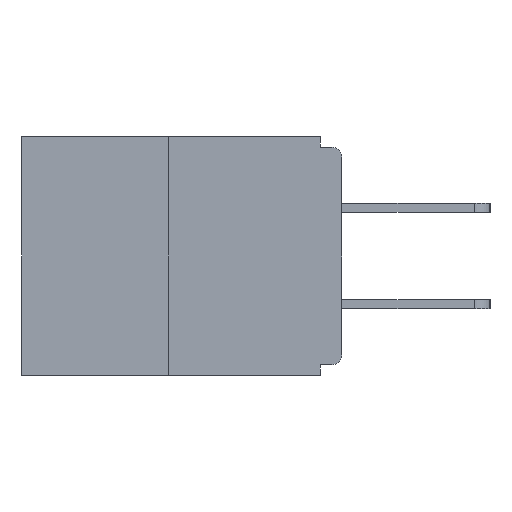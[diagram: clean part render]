
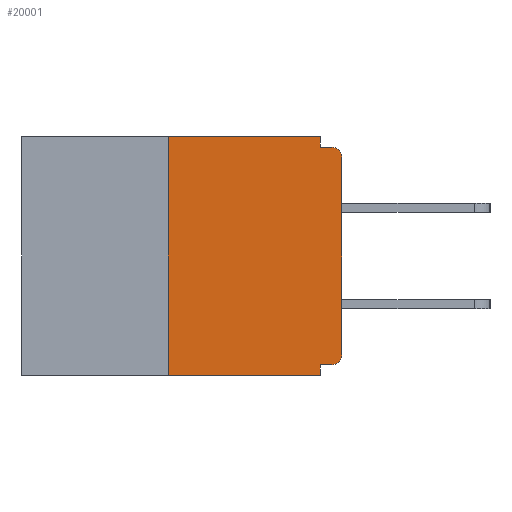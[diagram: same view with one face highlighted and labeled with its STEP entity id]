
A CAD part, left-side view. The second image highlights one B-rep face of the part: STEP entity #20001.
In plain terms, the highlighted planar face has unit normal (-1, 0, 0).
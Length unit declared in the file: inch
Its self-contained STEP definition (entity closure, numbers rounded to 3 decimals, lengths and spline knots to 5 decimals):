
#694 = CARTESIAN_POINT ( 'NONE',  ( 0., 0.031, -0.328 ) ) ;
#974 = CIRCLE ( 'NONE', #20030, 0.015 ) ;
#2123 = CARTESIAN_POINT ( 'NONE',  ( 0., 0., -0.03 ) ) ;
#2350 = LINE ( 'NONE', #13186, #14965 ) ;
#2419 = DIRECTION ( 'NONE',  ( 0., 0., 1. ) ) ;
#2422 = EDGE_CURVE ( 'NONE', #6759, #5591, #13960, .T. ) ;
#2708 = EDGE_CURVE ( 'NONE', #6008, #3499, #16280, .T. ) ;
#2768 = DIRECTION ( 'NONE',  ( 0., 0., 1. ) ) ;
#2793 = EDGE_CURVE ( 'NONE', #4504, #5591, #8411, .T. ) ;
#3046 = CARTESIAN_POINT ( 'NONE',  ( 0., 0., -0.313 ) ) ;
#3499 = VERTEX_POINT ( 'NONE', #15498 ) ;
#3586 = LINE ( 'NONE', #21746, #20382 ) ;
#3905 = CIRCLE ( 'NONE', #19775, 0.015 ) ;
#4391 = CARTESIAN_POINT ( 'NONE',  ( 0., 0.25, 0. ) ) ;
#4504 = VERTEX_POINT ( 'NONE', #14074 ) ;
#4991 = DIRECTION ( 'NONE',  ( 0., 0., -1. ) ) ;
#5195 = DIRECTION ( 'NONE',  ( 0., 0., -1. ) ) ;
#5329 = EDGE_CURVE ( 'NONE', #3499, #14498, #3586, .T. ) ;
#5591 = VERTEX_POINT ( 'NONE', #10942 ) ;
#5927 = AXIS2_PLACEMENT_3D ( 'NONE', #21095, #7773, #10938 ) ;
#6008 = VERTEX_POINT ( 'NONE', #6729 ) ;
#6123 = CARTESIAN_POINT ( 'NONE',  ( 0., 0.015, -0.015 ) ) ;
#6729 = CARTESIAN_POINT ( 'NONE',  ( 0., 0.25, 0. ) ) ;
#6759 = VERTEX_POINT ( 'NONE', #694 ) ;
#6825 = DIRECTION ( 'NONE',  ( 0., 0., -1. ) ) ;
#7468 = VERTEX_POINT ( 'NONE', #10617 ) ;
#7773 = DIRECTION ( 'NONE',  ( 1., 0., 0. ) ) ;
#7795 = CARTESIAN_POINT ( 'NONE',  ( 0., 0.015, -0.313 ) ) ;
#7820 = VERTEX_POINT ( 'NONE', #6123 ) ;
#8411 = LINE ( 'NONE', #15099, #11867 ) ;
#8590 = CARTESIAN_POINT ( 'NONE',  ( 0., 0.015, -0.03 ) ) ;
#8704 = VERTEX_POINT ( 'NONE', #2123 ) ;
#8822 = EDGE_CURVE ( 'NONE', #14498, #7820, #2350, .T. ) ;
#8902 = EDGE_CURVE ( 'NONE', #4504, #6008, #9736, .T. ) ;
#9533 = EDGE_CURVE ( 'NONE', #7468, #18814, #974, .T. ) ;
#9736 = LINE ( 'NONE', #4391, #16296 ) ;
#9774 = CARTESIAN_POINT ( 'NONE',  ( 0., 0.031, -0.015 ) ) ;
#9923 = EDGE_CURVE ( 'NONE', #18814, #8704, #11828, .T. ) ;
#10279 = DIRECTION ( 'NONE',  ( -1., 0., 0. ) ) ;
#10617 = CARTESIAN_POINT ( 'NONE',  ( 0., 0.015, -0.328 ) ) ;
#10938 = DIRECTION ( 'NONE',  ( 0., 0., -1. ) ) ;
#10942 = CARTESIAN_POINT ( 'NONE',  ( 0., 0.031, -0.343 ) ) ;
#11587 = ORIENTED_EDGE ( 'NONE', *, *, #8822, .F. ) ;
#11828 = LINE ( 'NONE', #20827, #21231 ) ;
#11867 = VECTOR ( 'NONE', #18313, 39.37008 ) ;
#11904 = ORIENTED_EDGE ( 'NONE', *, *, #17702, .T. ) ;
#13186 = CARTESIAN_POINT ( 'NONE',  ( 0., 0., -0.015 ) ) ;
#13726 = ORIENTED_EDGE ( 'NONE', *, *, #9923, .T. ) ;
#13960 = LINE ( 'NONE', #18189, #14972 ) ;
#14000 = VECTOR ( 'NONE', #20328, 39.37008 ) ;
#14074 = CARTESIAN_POINT ( 'NONE',  ( 0., 0.25, -0.343 ) ) ;
#14498 = VERTEX_POINT ( 'NONE', #9774 ) ;
#14740 = CARTESIAN_POINT ( 'NONE',  ( 0., 0.46, 0. ) ) ;
#14812 = DIRECTION ( 'NONE',  ( 0., -1., 0. ) ) ;
#14965 = VECTOR ( 'NONE', #18192, 39.37008 ) ;
#14972 = VECTOR ( 'NONE', #4991, 39.37008 ) ;
#15099 = CARTESIAN_POINT ( 'NONE',  ( 0., 0.46, -0.343 ) ) ;
#15498 = CARTESIAN_POINT ( 'NONE',  ( 0., 0.031, 0. ) ) ;
#15948 = DIRECTION ( 'NONE',  ( -1., 0., 0. ) ) ;
#16061 = PLANE ( 'NONE',  #5927 ) ;
#16280 = LINE ( 'NONE', #14740, #21260 ) ;
#16296 = VECTOR ( 'NONE', #2768, 39.37008 ) ;
#16445 = ORIENTED_EDGE ( 'NONE', *, *, #5329, .F. ) ;
#16863 = ORIENTED_EDGE ( 'NONE', *, *, #21469, .F. ) ;
#17202 = ORIENTED_EDGE ( 'NONE', *, *, #9533, .T. ) ;
#17702 = EDGE_CURVE ( 'NONE', #8704, #7820, #3905, .T. ) ;
#18189 = CARTESIAN_POINT ( 'NONE',  ( 0., 0.031, -0.343 ) ) ;
#18192 = DIRECTION ( 'NONE',  ( 0., -1., 0. ) ) ;
#18313 = DIRECTION ( 'NONE',  ( 0., -1., 0. ) ) ;
#18418 = LINE ( 'NONE', #18575, #14000 ) ;
#18575 = CARTESIAN_POINT ( 'NONE',  ( 0., 0., -0.328 ) ) ;
#18691 = ORIENTED_EDGE ( 'NONE', *, *, #8902, .F. ) ;
#18768 = ORIENTED_EDGE ( 'NONE', *, *, #2793, .T. ) ;
#18814 = VERTEX_POINT ( 'NONE', #3046 ) ;
#19582 = DIRECTION ( 'NONE',  ( 0., 0., -1. ) ) ;
#19775 = AXIS2_PLACEMENT_3D ( 'NONE', #8590, #10279, #6825 ) ;
#20001 = ADVANCED_FACE ( 'NONE', ( #21361 ), #16061, .F. ) ;
#20030 = AXIS2_PLACEMENT_3D ( 'NONE', #7795, #15948, #19582 ) ;
#20236 = ORIENTED_EDGE ( 'NONE', *, *, #2422, .F. ) ;
#20328 = DIRECTION ( 'NONE',  ( 0., 1., 0. ) ) ;
#20382 = VECTOR ( 'NONE', #5195, 39.37008 ) ;
#20542 = EDGE_LOOP ( 'NONE', ( #21725, #18691, #18768, #20236, #16863, #17202, #13726, #11904, #11587, #16445 ) ) ;
#20827 = CARTESIAN_POINT ( 'NONE',  ( 0., 0., 0. ) ) ;
#21095 = CARTESIAN_POINT ( 'NONE',  ( 0., 0.46, 0. ) ) ;
#21231 = VECTOR ( 'NONE', #2419, 39.37008 ) ;
#21260 = VECTOR ( 'NONE', #14812, 39.37008 ) ;
#21361 = FACE_OUTER_BOUND ( 'NONE', #20542, .T. ) ;
#21469 = EDGE_CURVE ( 'NONE', #7468, #6759, #18418, .T. ) ;
#21725 = ORIENTED_EDGE ( 'NONE', *, *, #2708, .F. ) ;
#21746 = CARTESIAN_POINT ( 'NONE',  ( 0., 0.031, 0. ) ) ;
